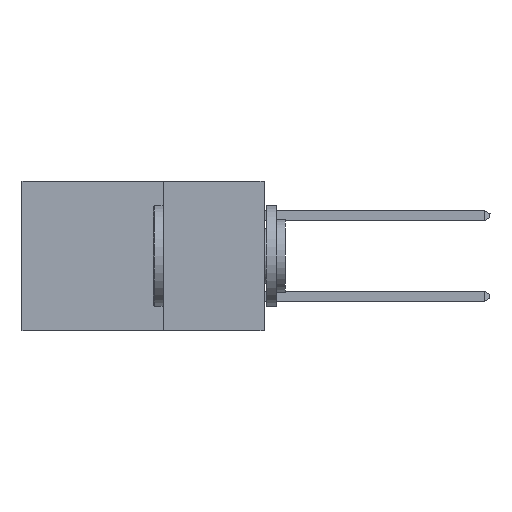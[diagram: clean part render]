
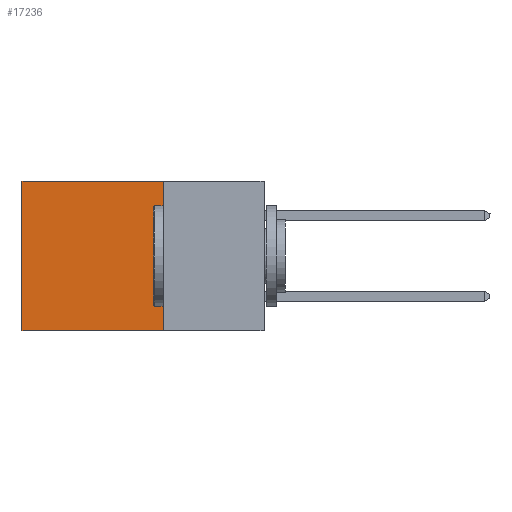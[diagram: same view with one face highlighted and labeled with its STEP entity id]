
A CAD part, left-side view. The second image highlights one B-rep face of the part: STEP entity #17236.
In plain terms, the highlighted planar face has unit normal (-1, 0, 0).
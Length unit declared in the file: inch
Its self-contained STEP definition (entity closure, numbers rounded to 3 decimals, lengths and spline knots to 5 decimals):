
#71 = DIRECTION ( 'NONE',  ( 1., 0., 0. ) ) ;
#1232 = AXIS2_PLACEMENT_3D ( 'NONE', #13389, #71, #18595 ) ;
#1270 = VECTOR ( 'NONE', #11770, 39.37008 ) ;
#1886 = CARTESIAN_POINT ( 'NONE',  ( 0.298, 0.25, -0.37 ) ) ;
#2905 = CARTESIAN_POINT ( 'NONE',  ( 0.298, 0.25, -0.37 ) ) ;
#4646 = VECTOR ( 'NONE', #33137, 39.37008 ) ;
#9069 = CARTESIAN_POINT ( 'NONE',  ( 0.298, 0.25, 0. ) ) ;
#9549 = VERTEX_POINT ( 'NONE', #2905 ) ;
#10325 = VERTEX_POINT ( 'NONE', #27196 ) ;
#11770 = DIRECTION ( 'NONE',  ( 0., 1., 0. ) ) ;
#12428 = DIRECTION ( 'NONE',  ( 0., 1., 0. ) ) ;
#12653 = EDGE_CURVE ( 'NONE', #13670, #9549, #25604, .T. ) ;
#13151 = EDGE_CURVE ( 'NONE', #10325, #19237, #30847, .T. ) ;
#13389 = CARTESIAN_POINT ( 'NONE',  ( 0.298, 0.25, 0. ) ) ;
#13670 = VERTEX_POINT ( 'NONE', #22196 ) ;
#13897 = FACE_OUTER_BOUND ( 'NONE', #21579, .T. ) ;
#15110 = CARTESIAN_POINT ( 'NONE',  ( 0.298, 0.6, 0. ) ) ;
#16798 = ORIENTED_EDGE ( 'NONE', *, *, #12653, .F. ) ;
#17065 = VECTOR ( 'NONE', #28036, 39.37008 ) ;
#17236 = ADVANCED_FACE ( 'NONE', ( #13897 ), #31513, .F. ) ;
#18294 = LINE ( 'NONE', #1886, #23535 ) ;
#18595 = DIRECTION ( 'NONE',  ( 0., 0., -1. ) ) ;
#19145 = CARTESIAN_POINT ( 'NONE',  ( 0.298, 0.6, -0.37 ) ) ;
#19237 = VERTEX_POINT ( 'NONE', #19145 ) ;
#20145 = CARTESIAN_POINT ( 'NONE',  ( 0.298, 0.25, 0. ) ) ;
#20597 = EDGE_CURVE ( 'NONE', #13670, #10325, #21865, .T. ) ;
#21579 = EDGE_LOOP ( 'NONE', ( #27824, #33860, #16798, #23123 ) ) ;
#21865 = LINE ( 'NONE', #9069, #1270 ) ;
#22196 = CARTESIAN_POINT ( 'NONE',  ( 0.298, 0.25, 0. ) ) ;
#23123 = ORIENTED_EDGE ( 'NONE', *, *, #20597, .T. ) ;
#23535 = VECTOR ( 'NONE', #12428, 39.37008 ) ;
#25604 = LINE ( 'NONE', #20145, #4646 ) ;
#26036 = EDGE_CURVE ( 'NONE', #9549, #19237, #18294, .T. ) ;
#27196 = CARTESIAN_POINT ( 'NONE',  ( 0.298, 0.6, 0. ) ) ;
#27824 = ORIENTED_EDGE ( 'NONE', *, *, #13151, .T. ) ;
#28036 = DIRECTION ( 'NONE',  ( 0., 0., -1. ) ) ;
#30847 = LINE ( 'NONE', #15110, #17065 ) ;
#31513 = PLANE ( 'NONE',  #1232 ) ;
#33137 = DIRECTION ( 'NONE',  ( 0., 0., -1. ) ) ;
#33860 = ORIENTED_EDGE ( 'NONE', *, *, #26036, .F. ) ;
